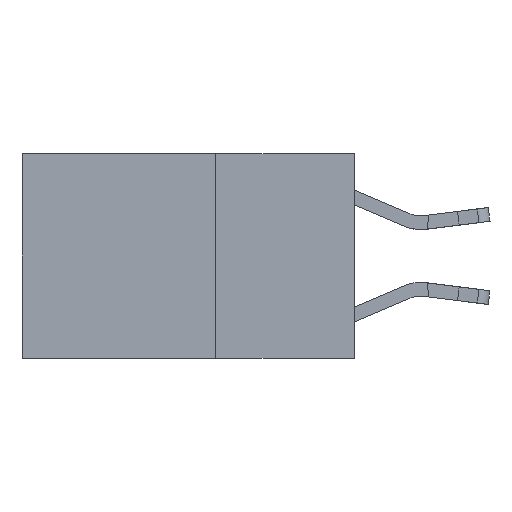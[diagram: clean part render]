
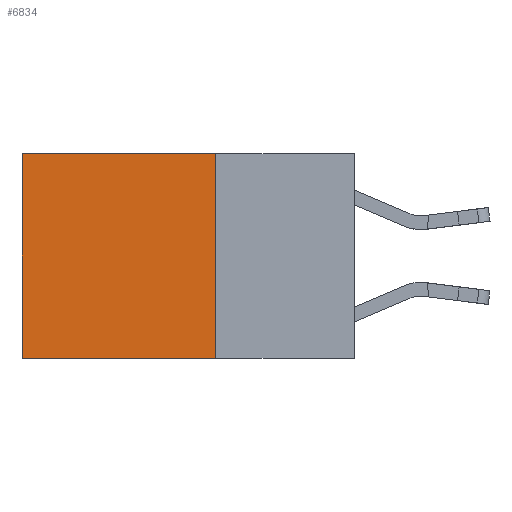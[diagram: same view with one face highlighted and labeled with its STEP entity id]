
A CAD part, left-side view. The second image highlights one B-rep face of the part: STEP entity #6834.
In plain terms, the highlighted planar face has unit normal (-1, 0, 0).
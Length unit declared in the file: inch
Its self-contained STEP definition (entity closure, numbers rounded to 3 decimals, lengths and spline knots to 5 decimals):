
#1651 = LINE ( 'NONE', #14316, #6359 ) ;
#1670 = CARTESIAN_POINT ( 'NONE',  ( 0.2625, 0.6, 0. ) ) ;
#1714 = AXIS2_PLACEMENT_3D ( 'NONE', #8581, #10336, #22462 ) ;
#2056 = DIRECTION ( 'NONE',  ( 0., 1., 0. ) ) ;
#2316 = EDGE_LOOP ( 'NONE', ( #2919, #15294, #15027, #18932 ) ) ;
#2481 = VECTOR ( 'NONE', #3803, 39.37008 ) ;
#2549 = DIRECTION ( 'NONE',  ( 0., 0., -1. ) ) ;
#2919 = ORIENTED_EDGE ( 'NONE', *, *, #13751, .T. ) ;
#3620 = CARTESIAN_POINT ( 'NONE',  ( 0.2625, 0.25, -0.37 ) ) ;
#3803 = DIRECTION ( 'NONE',  ( 0., 0., -1. ) ) ;
#4577 = CARTESIAN_POINT ( 'NONE',  ( 0.2625, 0.25, 0. ) ) ;
#5570 = CARTESIAN_POINT ( 'NONE',  ( 0.2625, 0.6, -0.37 ) ) ;
#6359 = VECTOR ( 'NONE', #2056, 39.37008 ) ;
#6834 = ADVANCED_FACE ( 'NONE', ( #20171 ), #19001, .F. ) ;
#7795 = CARTESIAN_POINT ( 'NONE',  ( 0.2625, 0.25, 0. ) ) ;
#8581 = CARTESIAN_POINT ( 'NONE',  ( 0.2625, 0.25, 0. ) ) ;
#8808 = LINE ( 'NONE', #21191, #2481 ) ;
#10336 = DIRECTION ( 'NONE',  ( 1., 0., 0. ) ) ;
#12696 = VECTOR ( 'NONE', #13970, 39.37008 ) ;
#13751 = EDGE_CURVE ( 'NONE', #20828, #19015, #8808, .T. ) ;
#13970 = DIRECTION ( 'NONE',  ( 0., 1., 0. ) ) ;
#14316 = CARTESIAN_POINT ( 'NONE',  ( 0.2625, 0.25, 0. ) ) ;
#15027 = ORIENTED_EDGE ( 'NONE', *, *, #16529, .F. ) ;
#15294 = ORIENTED_EDGE ( 'NONE', *, *, #16961, .F. ) ;
#16529 = EDGE_CURVE ( 'NONE', #16705, #17583, #17376, .T. ) ;
#16705 = VERTEX_POINT ( 'NONE', #4577 ) ;
#16961 = EDGE_CURVE ( 'NONE', #17583, #19015, #17350, .T. ) ;
#17350 = LINE ( 'NONE', #19131, #12696 ) ;
#17376 = LINE ( 'NONE', #7795, #22483 ) ;
#17583 = VERTEX_POINT ( 'NONE', #3620 ) ;
#18932 = ORIENTED_EDGE ( 'NONE', *, *, #20981, .T. ) ;
#19001 = PLANE ( 'NONE',  #1714 ) ;
#19015 = VERTEX_POINT ( 'NONE', #5570 ) ;
#19131 = CARTESIAN_POINT ( 'NONE',  ( 0.2625, 0.25, -0.37 ) ) ;
#20171 = FACE_OUTER_BOUND ( 'NONE', #2316, .T. ) ;
#20828 = VERTEX_POINT ( 'NONE', #1670 ) ;
#20981 = EDGE_CURVE ( 'NONE', #16705, #20828, #1651, .T. ) ;
#21191 = CARTESIAN_POINT ( 'NONE',  ( 0.2625, 0.6, 0. ) ) ;
#22462 = DIRECTION ( 'NONE',  ( 0., 0., -1. ) ) ;
#22483 = VECTOR ( 'NONE', #2549, 39.37008 ) ;
